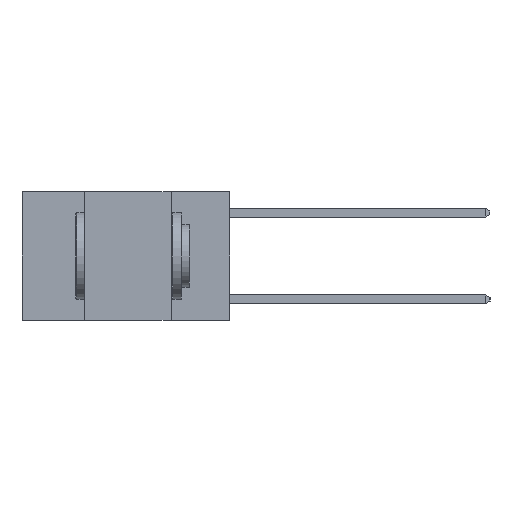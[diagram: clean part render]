
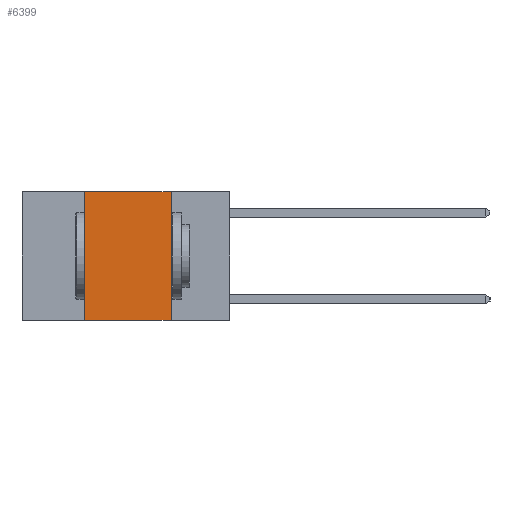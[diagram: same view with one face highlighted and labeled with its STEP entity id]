
A CAD part, left-side view. The second image highlights one B-rep face of the part: STEP entity #6399.
In plain terms, the highlighted planar face has unit normal (-1, 0, 0).
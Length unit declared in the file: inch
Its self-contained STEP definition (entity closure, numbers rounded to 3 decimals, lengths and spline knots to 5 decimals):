
#205 = CARTESIAN_POINT ( 'NONE',  ( 0., 0.42, 0. ) ) ;
#238 = CARTESIAN_POINT ( 'NONE',  ( 0., 0.42, 0. ) ) ;
#483 = CARTESIAN_POINT ( 'NONE',  ( 0., 0.42, -0.37 ) ) ;
#632 = AXIS2_PLACEMENT_3D ( 'NONE', #10131, #4906, #10948 ) ;
#959 = DIRECTION ( 'NONE',  ( 0., -1., 0. ) ) ;
#1128 = DIRECTION ( 'NONE',  ( 0., 0., 1. ) ) ;
#1719 = VECTOR ( 'NONE', #1128, 39.37008 ) ;
#1801 = DIRECTION ( 'NONE',  ( 0., -1., 0. ) ) ;
#2114 = FACE_OUTER_BOUND ( 'NONE', #8492, .T. ) ;
#2203 = VERTEX_POINT ( 'NONE', #7736 ) ;
#2403 = LINE ( 'NONE', #7080, #7008 ) ;
#2743 = VERTEX_POINT ( 'NONE', #483 ) ;
#3152 = LINE ( 'NONE', #4046, #5178 ) ;
#3169 = VERTEX_POINT ( 'NONE', #7305 ) ;
#3345 = EDGE_CURVE ( 'NONE', #7435, #2203, #3693, .T. ) ;
#3480 = ORIENTED_EDGE ( 'NONE', *, *, #5983, .T. ) ;
#3693 = LINE ( 'NONE', #5246, #8030 ) ;
#4046 = CARTESIAN_POINT ( 'NONE',  ( 0., 0.17, 0. ) ) ;
#4814 = EDGE_CURVE ( 'NONE', #2743, #7435, #8670, .T. ) ;
#4906 = DIRECTION ( 'NONE',  ( 1., 0., 0. ) ) ;
#5178 = VECTOR ( 'NONE', #8381, 39.37008 ) ;
#5246 = CARTESIAN_POINT ( 'NONE',  ( 0., 0.6, 0. ) ) ;
#5983 = EDGE_CURVE ( 'NONE', #2743, #3169, #2403, .T. ) ;
#6399 = ADVANCED_FACE ( 'NONE', ( #2114 ), #8387, .F. ) ;
#7008 = VECTOR ( 'NONE', #959, 39.37008 ) ;
#7080 = CARTESIAN_POINT ( 'NONE',  ( 0., 0.6, -0.37 ) ) ;
#7305 = CARTESIAN_POINT ( 'NONE',  ( 0., 0.17, -0.37 ) ) ;
#7435 = VERTEX_POINT ( 'NONE', #238 ) ;
#7736 = CARTESIAN_POINT ( 'NONE',  ( 0., 0.17, 0. ) ) ;
#8030 = VECTOR ( 'NONE', #1801, 39.37008 ) ;
#8381 = DIRECTION ( 'NONE',  ( 0., 0., -1. ) ) ;
#8387 = PLANE ( 'NONE',  #632 ) ;
#8492 = EDGE_LOOP ( 'NONE', ( #9160, #9491, #9761, #3480 ) ) ;
#8670 = LINE ( 'NONE', #205, #1719 ) ;
#9113 = EDGE_CURVE ( 'NONE', #2203, #3169, #3152, .T. ) ;
#9160 = ORIENTED_EDGE ( 'NONE', *, *, #9113, .F. ) ;
#9491 = ORIENTED_EDGE ( 'NONE', *, *, #3345, .F. ) ;
#9761 = ORIENTED_EDGE ( 'NONE', *, *, #4814, .F. ) ;
#10131 = CARTESIAN_POINT ( 'NONE',  ( 0., 0.6, 0. ) ) ;
#10948 = DIRECTION ( 'NONE',  ( 0., 0., -1. ) ) ;
